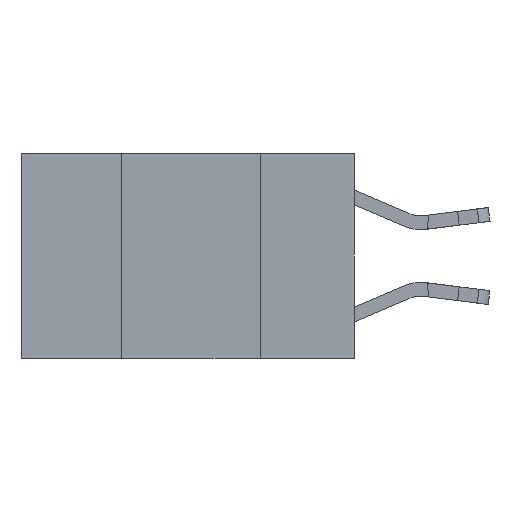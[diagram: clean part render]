
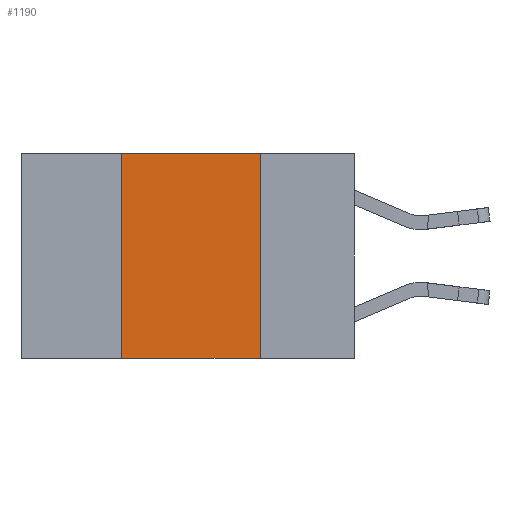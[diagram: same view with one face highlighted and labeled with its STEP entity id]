
A CAD part, left-side view. The second image highlights one B-rep face of the part: STEP entity #1190.
In plain terms, the highlighted planar face has unit normal (-1, 0, 0).
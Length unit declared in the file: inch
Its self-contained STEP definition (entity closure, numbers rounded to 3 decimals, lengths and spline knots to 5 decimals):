
#149 = EDGE_CURVE ( 'NONE', #987, #9892, #6079, .T. ) ;
#380 = PLANE ( 'NONE',  #8003 ) ;
#583 = VECTOR ( 'NONE', #5356, 39.37008 ) ;
#720 = CARTESIAN_POINT ( 'NONE',  ( 0., 0.6, -0.37 ) ) ;
#893 = CARTESIAN_POINT ( 'NONE',  ( 0., 0.42, -0.37 ) ) ;
#987 = VERTEX_POINT ( 'NONE', #893 ) ;
#1190 = ADVANCED_FACE ( 'NONE', ( #6590 ), #380, .F. ) ;
#1317 = VECTOR ( 'NONE', #3856, 39.37008 ) ;
#1364 = ORIENTED_EDGE ( 'NONE', *, *, #11921, .F. ) ;
#1755 = CARTESIAN_POINT ( 'NONE',  ( 0., 0.42, 0. ) ) ;
#2310 = CARTESIAN_POINT ( 'NONE',  ( 0., 0.17, -0.37 ) ) ;
#2747 = EDGE_CURVE ( 'NONE', #11240, #11995, #3750, .T. ) ;
#3486 = DIRECTION ( 'NONE',  ( 1., 0., 0. ) ) ;
#3750 = LINE ( 'NONE', #10222, #10480 ) ;
#3800 = ORIENTED_EDGE ( 'NONE', *, *, #149, .T. ) ;
#3856 = DIRECTION ( 'NONE',  ( 0., -1., 0. ) ) ;
#3924 = EDGE_LOOP ( 'NONE', ( #5881, #4431, #1364, #3800 ) ) ;
#3994 = LINE ( 'NONE', #1755, #13041 ) ;
#4431 = ORIENTED_EDGE ( 'NONE', *, *, #2747, .F. ) ;
#5356 = DIRECTION ( 'NONE',  ( 0., 0., -1. ) ) ;
#5881 = ORIENTED_EDGE ( 'NONE', *, *, #7795, .F. ) ;
#6079 = LINE ( 'NONE', #720, #1317 ) ;
#6590 = FACE_OUTER_BOUND ( 'NONE', #3924, .T. ) ;
#7110 = CARTESIAN_POINT ( 'NONE',  ( 0., 0.17, 0. ) ) ;
#7795 = EDGE_CURVE ( 'NONE', #11995, #9892, #12907, .T. ) ;
#8003 = AXIS2_PLACEMENT_3D ( 'NONE', #10636, #3486, #10709 ) ;
#8362 = CARTESIAN_POINT ( 'NONE',  ( 0., 0.42, 0. ) ) ;
#9892 = VERTEX_POINT ( 'NONE', #2310 ) ;
#10222 = CARTESIAN_POINT ( 'NONE',  ( 0., 0.6, 0. ) ) ;
#10480 = VECTOR ( 'NONE', #11135, 39.37008 ) ;
#10636 = CARTESIAN_POINT ( 'NONE',  ( 0., 0.6, 0. ) ) ;
#10709 = DIRECTION ( 'NONE',  ( 0., 0., -1. ) ) ;
#11135 = DIRECTION ( 'NONE',  ( 0., -1., 0. ) ) ;
#11240 = VERTEX_POINT ( 'NONE', #8362 ) ;
#11921 = EDGE_CURVE ( 'NONE', #987, #11240, #3994, .T. ) ;
#11995 = VERTEX_POINT ( 'NONE', #7110 ) ;
#12834 = CARTESIAN_POINT ( 'NONE',  ( 0., 0.17, 0. ) ) ;
#12907 = LINE ( 'NONE', #12834, #583 ) ;
#13041 = VECTOR ( 'NONE', #13373, 39.37008 ) ;
#13373 = DIRECTION ( 'NONE',  ( 0., 0., 1. ) ) ;
